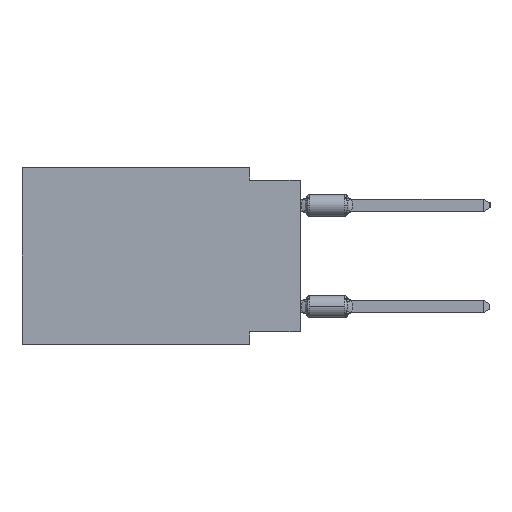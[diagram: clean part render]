
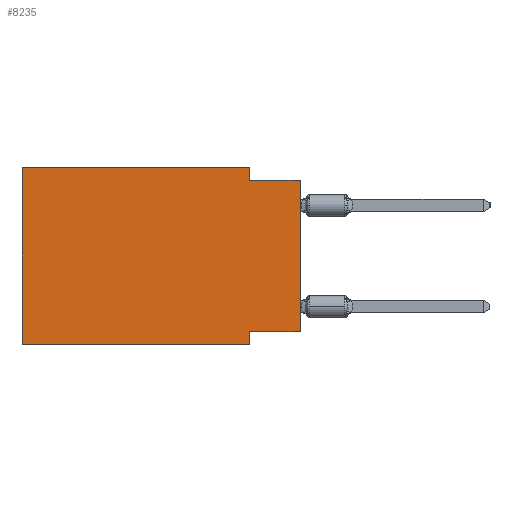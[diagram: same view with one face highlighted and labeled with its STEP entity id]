
A CAD part, left-side view. The second image highlights one B-rep face of the part: STEP entity #8235.
In plain terms, the highlighted planar face has unit normal (-1, 0, 0).
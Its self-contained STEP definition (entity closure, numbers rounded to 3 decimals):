
#1270 = VERTEX_POINT ( 'NONE', #18176 ) ;
#1452 = EDGE_CURVE ( 'NONE', #3732, #30694, #22624, .T. ) ;
#2619 = ORIENTED_EDGE ( 'NONE', *, *, #34857, .F. ) ;
#2648 = CARTESIAN_POINT ( 'NONE',  ( 0., 0., 0. ) ) ;
#3732 = VERTEX_POINT ( 'NONE', #19541 ) ;
#3919 = DIRECTION ( 'NONE',  ( 0., -1., 0. ) ) ;
#4927 = CARTESIAN_POINT ( 'NONE',  ( 0., 0., -8.255 ) ) ;
#5037 = VECTOR ( 'NONE', #32381, 1000. ) ;
#5985 = LINE ( 'NONE', #23242, #25687 ) ;
#6885 = CARTESIAN_POINT ( 'NONE',  ( 0., 0., -8.255 ) ) ;
#7242 = AXIS2_PLACEMENT_3D ( 'NONE', #33626, #8230, #16062 ) ;
#8230 = DIRECTION ( 'NONE',  ( 1., 0., 0. ) ) ;
#8235 = ADVANCED_FACE ( 'NONE', ( #13640 ), #22355, .F. ) ;
#8489 = CARTESIAN_POINT ( 'NONE',  ( 0., 2.54, 0. ) ) ;
#8902 = CARTESIAN_POINT ( 'NONE',  ( 0., 13.97, -8.89 ) ) ;
#9982 = EDGE_CURVE ( 'NONE', #27735, #10888, #14498, .T. ) ;
#10136 = CARTESIAN_POINT ( 'NONE',  ( 0., 2.54, -0.635 ) ) ;
#10888 = VERTEX_POINT ( 'NONE', #21038 ) ;
#10916 = VECTOR ( 'NONE', #16046, 1000. ) ;
#12578 = VERTEX_POINT ( 'NONE', #31422 ) ;
#13640 = FACE_OUTER_BOUND ( 'NONE', #14389, .T. ) ;
#14018 = EDGE_CURVE ( 'NONE', #18345, #1270, #22515, .T. ) ;
#14371 = ORIENTED_EDGE ( 'NONE', *, *, #28863, .F. ) ;
#14389 = EDGE_LOOP ( 'NONE', ( #33646, #14371, #29841, #28176, #19556, #31102, #30745, #2619 ) ) ;
#14498 = LINE ( 'NONE', #33947, #33565 ) ;
#15953 = CARTESIAN_POINT ( 'NONE',  ( 0., 13.97, 0. ) ) ;
#16046 = DIRECTION ( 'NONE',  ( 0., 0., 1. ) ) ;
#16062 = DIRECTION ( 'NONE',  ( 0., 0., -1. ) ) ;
#16390 = DIRECTION ( 'NONE',  ( 0., 0., 1. ) ) ;
#16774 = CARTESIAN_POINT ( 'NONE',  ( 0., 13.97, -8.89 ) ) ;
#17666 = CARTESIAN_POINT ( 'NONE',  ( 0., 2.54, -8.255 ) ) ;
#18176 = CARTESIAN_POINT ( 'NONE',  ( 0., 13.97, 0. ) ) ;
#18345 = VERTEX_POINT ( 'NONE', #16774 ) ;
#18414 = DIRECTION ( 'NONE',  ( 0., 1., 0. ) ) ;
#19541 = CARTESIAN_POINT ( 'NONE',  ( 0., 2.54, 0. ) ) ;
#19556 = ORIENTED_EDGE ( 'NONE', *, *, #14018, .F. ) ;
#21038 = CARTESIAN_POINT ( 'NONE',  ( 0., 2.54, -8.89 ) ) ;
#22355 = PLANE ( 'NONE',  #7242 ) ;
#22515 = LINE ( 'NONE', #33784, #36159 ) ;
#22624 = LINE ( 'NONE', #8489, #27104 ) ;
#23242 = CARTESIAN_POINT ( 'NONE',  ( 0., 0., -0.635 ) ) ;
#25119 = LINE ( 'NONE', #2648, #10916 ) ;
#25665 = VERTEX_POINT ( 'NONE', #4927 ) ;
#25687 = VECTOR ( 'NONE', #3919, 1000. ) ;
#25827 = DIRECTION ( 'NONE',  ( 0., 0., -1. ) ) ;
#25981 = EDGE_CURVE ( 'NONE', #25665, #12578, #25119, .T. ) ;
#26900 = DIRECTION ( 'NONE',  ( 0., -1., 0. ) ) ;
#27104 = VECTOR ( 'NONE', #31664, 1000. ) ;
#27735 = VERTEX_POINT ( 'NONE', #17666 ) ;
#28065 = EDGE_CURVE ( 'NONE', #18345, #10888, #34977, .T. ) ;
#28176 = ORIENTED_EDGE ( 'NONE', *, *, #29373, .F. ) ;
#28863 = EDGE_CURVE ( 'NONE', #30694, #12578, #5985, .T. ) ;
#29373 = EDGE_CURVE ( 'NONE', #1270, #3732, #35583, .T. ) ;
#29841 = ORIENTED_EDGE ( 'NONE', *, *, #1452, .F. ) ;
#29852 = VECTOR ( 'NONE', #26900, 1000. ) ;
#30694 = VERTEX_POINT ( 'NONE', #10136 ) ;
#30745 = ORIENTED_EDGE ( 'NONE', *, *, #9982, .F. ) ;
#31102 = ORIENTED_EDGE ( 'NONE', *, *, #28065, .T. ) ;
#31422 = CARTESIAN_POINT ( 'NONE',  ( 0., 0., -0.635 ) ) ;
#31664 = DIRECTION ( 'NONE',  ( 0., 0., -1. ) ) ;
#32381 = DIRECTION ( 'NONE',  ( 0., -1., 0. ) ) ;
#33565 = VECTOR ( 'NONE', #25827, 1000. ) ;
#33626 = CARTESIAN_POINT ( 'NONE',  ( 0., 13.97, 0. ) ) ;
#33646 = ORIENTED_EDGE ( 'NONE', *, *, #25981, .T. ) ;
#33784 = CARTESIAN_POINT ( 'NONE',  ( 0., 13.97, 0. ) ) ;
#33947 = CARTESIAN_POINT ( 'NONE',  ( 0., 2.54, -8.89 ) ) ;
#34857 = EDGE_CURVE ( 'NONE', #25665, #27735, #35243, .T. ) ;
#34977 = LINE ( 'NONE', #8902, #5037 ) ;
#35243 = LINE ( 'NONE', #6885, #36008 ) ;
#35583 = LINE ( 'NONE', #15953, #29852 ) ;
#36008 = VECTOR ( 'NONE', #18414, 1000. ) ;
#36159 = VECTOR ( 'NONE', #16390, 1000. ) ;
